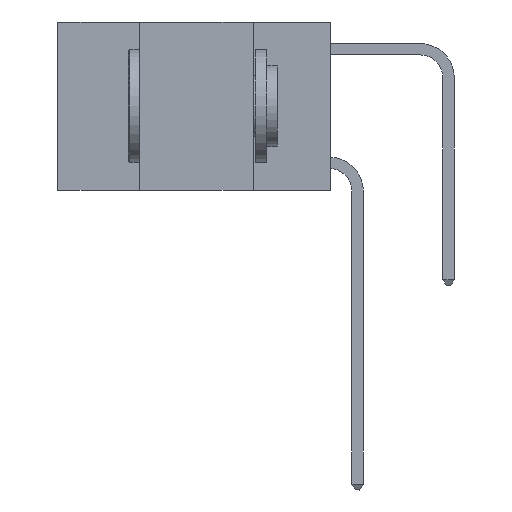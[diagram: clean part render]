
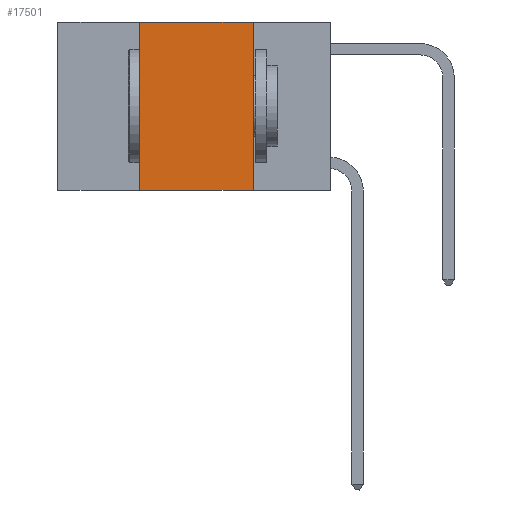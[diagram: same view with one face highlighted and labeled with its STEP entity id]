
A CAD part, left-side view. The second image highlights one B-rep face of the part: STEP entity #17501.
In plain terms, the highlighted planar face has unit normal (-1, 0, 0).
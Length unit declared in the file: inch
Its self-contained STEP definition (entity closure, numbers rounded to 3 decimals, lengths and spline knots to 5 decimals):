
#107 = ORIENTED_EDGE ( 'NONE', *, *, #21368, .F. ) ;
#2394 = EDGE_CURVE ( 'NONE', #5094, #18030, #18926, .T. ) ;
#3313 = ORIENTED_EDGE ( 'NONE', *, *, #2394, .F. ) ;
#3320 = VECTOR ( 'NONE', #15285, 39.37008 ) ;
#4269 = DIRECTION ( 'NONE',  ( 0., 0., -1. ) ) ;
#4515 = DIRECTION ( 'NONE',  ( 0., -1., 0. ) ) ;
#5094 = VERTEX_POINT ( 'NONE', #10745 ) ;
#7599 = CARTESIAN_POINT ( 'NONE',  ( 0., 0.42, 0. ) ) ;
#8497 = CARTESIAN_POINT ( 'NONE',  ( 0., 0.17, 0. ) ) ;
#8657 = VECTOR ( 'NONE', #4515, 39.37008 ) ;
#9100 = LINE ( 'NONE', #15046, #25639 ) ;
#10349 = VECTOR ( 'NONE', #17635, 39.37008 ) ;
#10745 = CARTESIAN_POINT ( 'NONE',  ( 0., 0.42, -0.37 ) ) ;
#11725 = CARTESIAN_POINT ( 'NONE',  ( 0., 0.17, -0.37 ) ) ;
#12594 = AXIS2_PLACEMENT_3D ( 'NONE', #13108, #27814, #15194 ) ;
#13108 = CARTESIAN_POINT ( 'NONE',  ( 0., 0.6, 0. ) ) ;
#14176 = EDGE_LOOP ( 'NONE', ( #107, #25381, #3313, #19959 ) ) ;
#15046 = CARTESIAN_POINT ( 'NONE',  ( 0., 0.17, 0. ) ) ;
#15194 = DIRECTION ( 'NONE',  ( 0., 0., -1. ) ) ;
#15277 = CARTESIAN_POINT ( 'NONE',  ( 0., 0.6, -0.37 ) ) ;
#15285 = DIRECTION ( 'NONE',  ( 0., 0., 1. ) ) ;
#17113 = PLANE ( 'NONE',  #12594 ) ;
#17126 = LINE ( 'NONE', #19616, #10349 ) ;
#17501 = ADVANCED_FACE ( 'NONE', ( #17799 ), #17113, .F. ) ;
#17548 = EDGE_CURVE ( 'NONE', #5094, #21668, #20129, .T. ) ;
#17635 = DIRECTION ( 'NONE',  ( 0., -1., 0. ) ) ;
#17799 = FACE_OUTER_BOUND ( 'NONE', #14176, .T. ) ;
#17874 = CARTESIAN_POINT ( 'NONE',  ( 0., 0.42, 0. ) ) ;
#18030 = VERTEX_POINT ( 'NONE', #7599 ) ;
#18926 = LINE ( 'NONE', #17874, #3320 ) ;
#19616 = CARTESIAN_POINT ( 'NONE',  ( 0., 0.6, 0. ) ) ;
#19959 = ORIENTED_EDGE ( 'NONE', *, *, #17548, .T. ) ;
#20059 = VERTEX_POINT ( 'NONE', #8497 ) ;
#20129 = LINE ( 'NONE', #15277, #8657 ) ;
#21368 = EDGE_CURVE ( 'NONE', #20059, #21668, #9100, .T. ) ;
#21668 = VERTEX_POINT ( 'NONE', #11725 ) ;
#23620 = EDGE_CURVE ( 'NONE', #18030, #20059, #17126, .T. ) ;
#25381 = ORIENTED_EDGE ( 'NONE', *, *, #23620, .F. ) ;
#25639 = VECTOR ( 'NONE', #4269, 39.37008 ) ;
#27814 = DIRECTION ( 'NONE',  ( 1., 0., 0. ) ) ;
